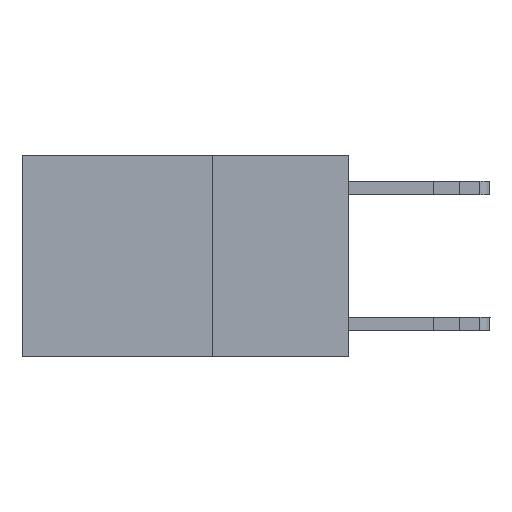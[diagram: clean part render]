
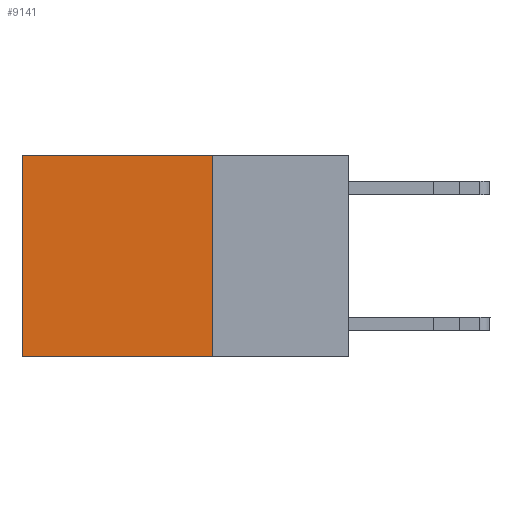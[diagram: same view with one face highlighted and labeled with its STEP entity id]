
A CAD part, left-side view. The second image highlights one B-rep face of the part: STEP entity #9141.
In plain terms, the highlighted planar face has unit normal (-1, 0, 0).
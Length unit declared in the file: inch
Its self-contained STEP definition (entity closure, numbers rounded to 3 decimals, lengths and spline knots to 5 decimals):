
#308 = CARTESIAN_POINT ( 'NONE',  ( 0.2625, 0.25, 0. ) ) ;
#2442 = VECTOR ( 'NONE', #8794, 39.37008 ) ;
#2566 = LINE ( 'NONE', #8407, #2442 ) ;
#2708 = EDGE_CURVE ( 'NONE', #3516, #20124, #3827, .T. ) ;
#3516 = VERTEX_POINT ( 'NONE', #16813 ) ;
#3827 = LINE ( 'NONE', #4581, #4062 ) ;
#3912 = FACE_OUTER_BOUND ( 'NONE', #18879, .T. ) ;
#4062 = VECTOR ( 'NONE', #4654, 39.37008 ) ;
#4457 = EDGE_CURVE ( 'NONE', #15927, #10534, #2566, .T. ) ;
#4581 = CARTESIAN_POINT ( 'NONE',  ( 0.2625, 0.25, -0.37 ) ) ;
#4654 = DIRECTION ( 'NONE',  ( 0., 1., 0. ) ) ;
#4971 = ORIENTED_EDGE ( 'NONE', *, *, #12065, .F. ) ;
#8407 = CARTESIAN_POINT ( 'NONE',  ( 0.2625, 0.25, 0. ) ) ;
#8794 = DIRECTION ( 'NONE',  ( 0., 1., 0. ) ) ;
#9141 = ADVANCED_FACE ( 'NONE', ( #3912 ), #20074, .F. ) ;
#9333 = ORIENTED_EDGE ( 'NONE', *, *, #2708, .F. ) ;
#10534 = VERTEX_POINT ( 'NONE', #13630 ) ;
#12065 = EDGE_CURVE ( 'NONE', #15927, #3516, #15196, .T. ) ;
#12296 = CARTESIAN_POINT ( 'NONE',  ( 0.2625, 0.6, -0.37 ) ) ;
#13040 = ORIENTED_EDGE ( 'NONE', *, *, #4457, .T. ) ;
#13245 = AXIS2_PLACEMENT_3D ( 'NONE', #19894, #19723, #19679 ) ;
#13630 = CARTESIAN_POINT ( 'NONE',  ( 0.2625, 0.6, 0. ) ) ;
#14172 = CARTESIAN_POINT ( 'NONE',  ( 0.2625, 0.6, 0. ) ) ;
#14426 = DIRECTION ( 'NONE',  ( 0., 0., -1. ) ) ;
#15196 = LINE ( 'NONE', #16311, #15517 ) ;
#15517 = VECTOR ( 'NONE', #16396, 39.37008 ) ;
#15927 = VERTEX_POINT ( 'NONE', #308 ) ;
#16311 = CARTESIAN_POINT ( 'NONE',  ( 0.2625, 0.25, 0. ) ) ;
#16396 = DIRECTION ( 'NONE',  ( 0., 0., -1. ) ) ;
#16440 = ORIENTED_EDGE ( 'NONE', *, *, #17499, .T. ) ;
#16813 = CARTESIAN_POINT ( 'NONE',  ( 0.2625, 0.25, -0.37 ) ) ;
#17499 = EDGE_CURVE ( 'NONE', #10534, #20124, #17704, .T. ) ;
#17704 = LINE ( 'NONE', #14172, #18476 ) ;
#18476 = VECTOR ( 'NONE', #14426, 39.37008 ) ;
#18879 = EDGE_LOOP ( 'NONE', ( #16440, #9333, #4971, #13040 ) ) ;
#19679 = DIRECTION ( 'NONE',  ( 0., 0., -1. ) ) ;
#19723 = DIRECTION ( 'NONE',  ( 1., 0., 0. ) ) ;
#19894 = CARTESIAN_POINT ( 'NONE',  ( 0.2625, 0.25, 0. ) ) ;
#20074 = PLANE ( 'NONE',  #13245 ) ;
#20124 = VERTEX_POINT ( 'NONE', #12296 ) ;
